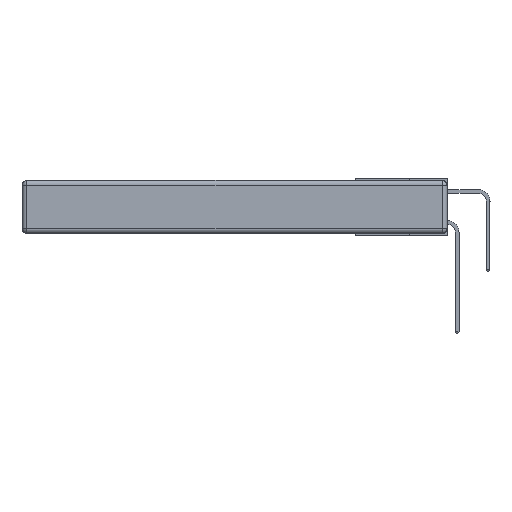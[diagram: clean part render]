
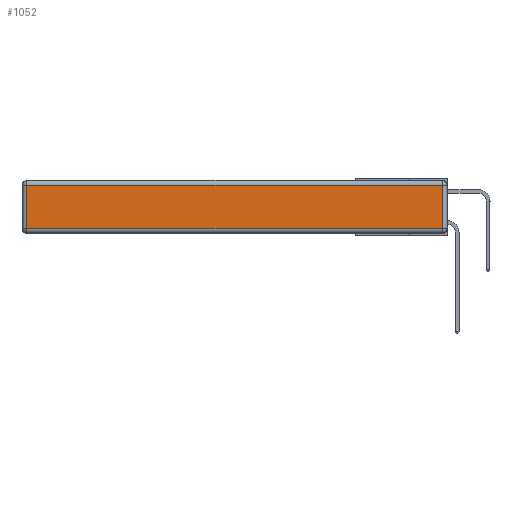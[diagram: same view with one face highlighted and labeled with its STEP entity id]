
A CAD part, left-side view. The second image highlights one B-rep face of the part: STEP entity #1052.
In plain terms, the highlighted planar face has unit normal (-1, 0, 0).
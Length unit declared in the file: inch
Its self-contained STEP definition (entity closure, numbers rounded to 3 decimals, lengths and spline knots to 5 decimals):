
#52 = CARTESIAN_POINT ( 'NONE',  ( 0., 2.72, -0.343 ) ) ;
#414 = VERTEX_POINT ( 'NONE', #5065 ) ;
#855 = DIRECTION ( 'NONE',  ( 0., -1., 0. ) ) ;
#1052 = ADVANCED_FACE ( 'NONE', ( #10502 ), #5369, .T. ) ;
#1682 = VERTEX_POINT ( 'NONE', #24442 ) ;
#2134 = EDGE_CURVE ( 'NONE', #8265, #414, #20087, .T. ) ;
#3548 = VERTEX_POINT ( 'NONE', #4435 ) ;
#3792 = CARTESIAN_POINT ( 'NONE',  ( 0., 0.03, -0.03 ) ) ;
#3937 = EDGE_CURVE ( 'NONE', #414, #3548, #4695, .T. ) ;
#4125 = CARTESIAN_POINT ( 'NONE',  ( 0., 0.03, -0.343 ) ) ;
#4435 = CARTESIAN_POINT ( 'NONE',  ( 0., 2.72, -0.313 ) ) ;
#4578 = LINE ( 'NONE', #4125, #24400 ) ;
#4695 = LINE ( 'NONE', #52, #15815 ) ;
#5065 = CARTESIAN_POINT ( 'NONE',  ( 0., 2.72, -0.03 ) ) ;
#5369 = PLANE ( 'NONE',  #6810 ) ;
#6810 = AXIS2_PLACEMENT_3D ( 'NONE', #24787, #13127, #7457 ) ;
#7318 = EDGE_LOOP ( 'NONE', ( #21720, #14649, #14525, #21487 ) ) ;
#7457 = DIRECTION ( 'NONE',  ( 0., 0., 1. ) ) ;
#7758 = EDGE_CURVE ( 'NONE', #1682, #8265, #4578, .T. ) ;
#8265 = VERTEX_POINT ( 'NONE', #3792 ) ;
#10502 = FACE_OUTER_BOUND ( 'NONE', #7318, .T. ) ;
#11637 = DIRECTION ( 'NONE',  ( 0., 0., -1. ) ) ;
#12250 = LINE ( 'NONE', #12363, #15875 ) ;
#12363 = CARTESIAN_POINT ( 'NONE',  ( 0., 0., -0.313 ) ) ;
#13127 = DIRECTION ( 'NONE',  ( -1., 0., 0. ) ) ;
#14525 = ORIENTED_EDGE ( 'NONE', *, *, #2134, .T. ) ;
#14649 = ORIENTED_EDGE ( 'NONE', *, *, #7758, .T. ) ;
#15815 = VECTOR ( 'NONE', #11637, 39.37008 ) ;
#15875 = VECTOR ( 'NONE', #855, 39.37008 ) ;
#18973 = CARTESIAN_POINT ( 'NONE',  ( 0., 2.75, -0.03 ) ) ;
#19212 = VECTOR ( 'NONE', #20651, 39.37008 ) ;
#20087 = LINE ( 'NONE', #18973, #19212 ) ;
#20638 = EDGE_CURVE ( 'NONE', #3548, #1682, #12250, .T. ) ;
#20651 = DIRECTION ( 'NONE',  ( 0., 1., 0. ) ) ;
#21487 = ORIENTED_EDGE ( 'NONE', *, *, #3937, .T. ) ;
#21720 = ORIENTED_EDGE ( 'NONE', *, *, #20638, .T. ) ;
#23206 = DIRECTION ( 'NONE',  ( 0., 0., 1. ) ) ;
#24400 = VECTOR ( 'NONE', #23206, 39.37008 ) ;
#24442 = CARTESIAN_POINT ( 'NONE',  ( 0., 0.03, -0.313 ) ) ;
#24787 = CARTESIAN_POINT ( 'NONE',  ( 0., 0., -0.343 ) ) ;
